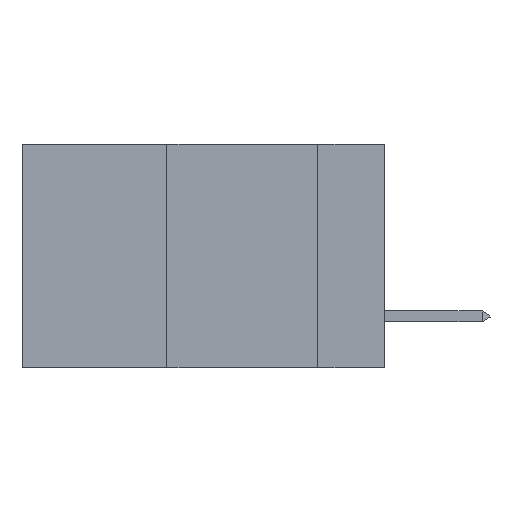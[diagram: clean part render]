
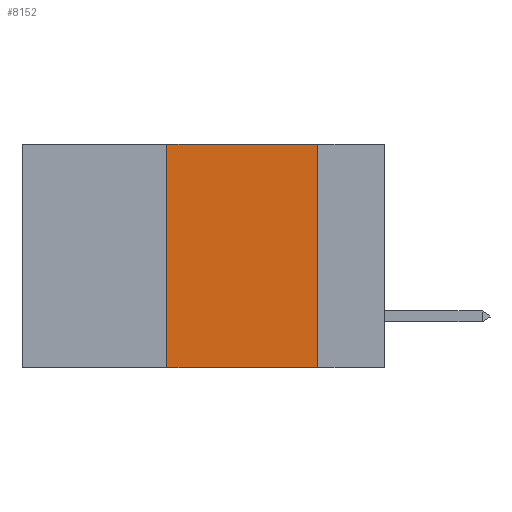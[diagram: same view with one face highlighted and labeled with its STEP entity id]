
A CAD part, left-side view. The second image highlights one B-rep face of the part: STEP entity #8152.
In plain terms, the highlighted planar face has unit normal (-1, 0, 0).
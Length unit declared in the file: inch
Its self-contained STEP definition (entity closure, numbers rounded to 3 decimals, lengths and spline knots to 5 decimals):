
#313 = VECTOR ( 'NONE', #13575, 39.37008 ) ;
#333 = VECTOR ( 'NONE', #9562, 39.37008 ) ;
#518 = EDGE_LOOP ( 'NONE', ( #16730, #2706, #17055, #9635 ) ) ;
#833 = FACE_OUTER_BOUND ( 'NONE', #518, .T. ) ;
#940 = VERTEX_POINT ( 'NONE', #16616 ) ;
#1212 = CARTESIAN_POINT ( 'NONE',  ( 0., 0.11, -0.37 ) ) ;
#1531 = EDGE_CURVE ( 'NONE', #4545, #7228, #19406, .T. ) ;
#1616 = CARTESIAN_POINT ( 'NONE',  ( 0., 0.6, 0. ) ) ;
#1853 = VECTOR ( 'NONE', #17691, 39.37008 ) ;
#2240 = LINE ( 'NONE', #17221, #333 ) ;
#2706 = ORIENTED_EDGE ( 'NONE', *, *, #7978, .F. ) ;
#4545 = VERTEX_POINT ( 'NONE', #9650 ) ;
#5644 = LINE ( 'NONE', #7371, #11021 ) ;
#5797 = EDGE_CURVE ( 'NONE', #940, #7228, #5644, .T. ) ;
#6418 = EDGE_CURVE ( 'NONE', #4545, #7322, #7022, .T. ) ;
#7022 = LINE ( 'NONE', #16199, #1853 ) ;
#7228 = VERTEX_POINT ( 'NONE', #1212 ) ;
#7322 = VERTEX_POINT ( 'NONE', #14978 ) ;
#7371 = CARTESIAN_POINT ( 'NONE',  ( 0., 0.11, 0. ) ) ;
#7978 = EDGE_CURVE ( 'NONE', #7322, #940, #2240, .T. ) ;
#8152 = ADVANCED_FACE ( 'NONE', ( #833 ), #8948, .F. ) ;
#8884 = DIRECTION ( 'NONE',  ( 0., 0., -1. ) ) ;
#8948 = PLANE ( 'NONE',  #13798 ) ;
#9143 = DIRECTION ( 'NONE',  ( 1., 0., 0. ) ) ;
#9562 = DIRECTION ( 'NONE',  ( 0., -1., 0. ) ) ;
#9635 = ORIENTED_EDGE ( 'NONE', *, *, #1531, .T. ) ;
#9650 = CARTESIAN_POINT ( 'NONE',  ( 0., 0.36, -0.37 ) ) ;
#10449 = DIRECTION ( 'NONE',  ( 0., 0., -1. ) ) ;
#11021 = VECTOR ( 'NONE', #8884, 39.37008 ) ;
#11913 = CARTESIAN_POINT ( 'NONE',  ( 0., 0.6, -0.37 ) ) ;
#13575 = DIRECTION ( 'NONE',  ( 0., -1., 0. ) ) ;
#13798 = AXIS2_PLACEMENT_3D ( 'NONE', #1616, #9143, #10449 ) ;
#14978 = CARTESIAN_POINT ( 'NONE',  ( 0., 0.36, 0. ) ) ;
#16199 = CARTESIAN_POINT ( 'NONE',  ( 0., 0.36, 0. ) ) ;
#16616 = CARTESIAN_POINT ( 'NONE',  ( 0., 0.11, 0. ) ) ;
#16730 = ORIENTED_EDGE ( 'NONE', *, *, #5797, .F. ) ;
#17055 = ORIENTED_EDGE ( 'NONE', *, *, #6418, .F. ) ;
#17221 = CARTESIAN_POINT ( 'NONE',  ( 0., 0.6, 0. ) ) ;
#17691 = DIRECTION ( 'NONE',  ( 0., 0., 1. ) ) ;
#19406 = LINE ( 'NONE', #11913, #313 ) ;
